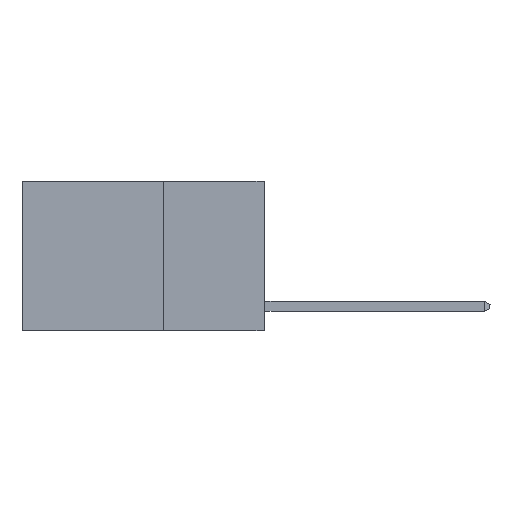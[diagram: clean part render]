
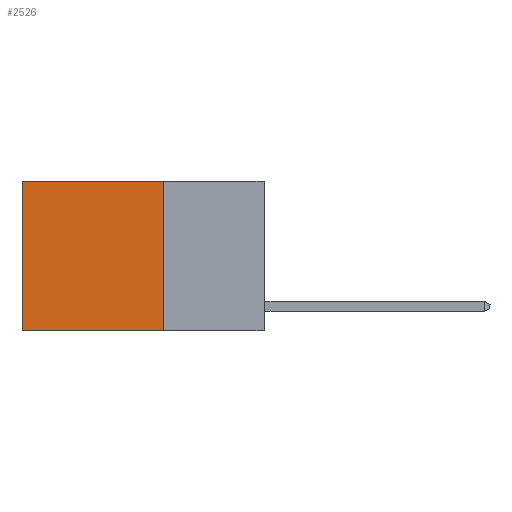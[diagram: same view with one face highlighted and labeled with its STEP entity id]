
A CAD part, left-side view. The second image highlights one B-rep face of the part: STEP entity #2526.
In plain terms, the highlighted planar face has unit normal (-1, 0, 0).
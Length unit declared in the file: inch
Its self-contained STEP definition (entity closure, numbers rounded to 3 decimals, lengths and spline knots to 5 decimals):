
#67 = PLANE ( 'NONE',  #14934 ) ;
#180 = VECTOR ( 'NONE', #2804, 39.37008 ) ;
#997 = CARTESIAN_POINT ( 'NONE',  ( 0.2625, 0.25, 0. ) ) ;
#2526 = ADVANCED_FACE ( 'NONE', ( #22917 ), #67, .F. ) ;
#2804 = DIRECTION ( 'NONE',  ( 0., 0., -1. ) ) ;
#2872 = ORIENTED_EDGE ( 'NONE', *, *, #22839, .F. ) ;
#3686 = DIRECTION ( 'NONE',  ( 0., 0., -1. ) ) ;
#4414 = CARTESIAN_POINT ( 'NONE',  ( 0.2625, 0.6, -0.37 ) ) ;
#4591 = EDGE_LOOP ( 'NONE', ( #13595, #2872, #7528, #22480 ) ) ;
#4717 = CARTESIAN_POINT ( 'NONE',  ( 0.2625, 0.25, -0.37 ) ) ;
#4904 = VECTOR ( 'NONE', #19980, 39.37008 ) ;
#5518 = LINE ( 'NONE', #997, #180 ) ;
#5565 = VECTOR ( 'NONE', #17342, 39.37008 ) ;
#6253 = LINE ( 'NONE', #21526, #19603 ) ;
#6656 = EDGE_CURVE ( 'NONE', #20534, #10073, #15682, .T. ) ;
#7018 = DIRECTION ( 'NONE',  ( 0., 0., -1. ) ) ;
#7486 = VERTEX_POINT ( 'NONE', #4414 ) ;
#7528 = ORIENTED_EDGE ( 'NONE', *, *, #12816, .F. ) ;
#9021 = CARTESIAN_POINT ( 'NONE',  ( 0.2625, 0.25, -0.37 ) ) ;
#9316 = EDGE_CURVE ( 'NONE', #10073, #7486, #6253, .T. ) ;
#10073 = VERTEX_POINT ( 'NONE', #21808 ) ;
#12684 = CARTESIAN_POINT ( 'NONE',  ( 0.2625, 0.25, 0. ) ) ;
#12816 = EDGE_CURVE ( 'NONE', #20534, #14226, #5518, .T. ) ;
#13595 = ORIENTED_EDGE ( 'NONE', *, *, #9316, .T. ) ;
#14226 = VERTEX_POINT ( 'NONE', #9021 ) ;
#14516 = DIRECTION ( 'NONE',  ( 1., 0., 0. ) ) ;
#14545 = CARTESIAN_POINT ( 'NONE',  ( 0.2625, 0.25, 0. ) ) ;
#14934 = AXIS2_PLACEMENT_3D ( 'NONE', #12684, #14516, #3686 ) ;
#15682 = LINE ( 'NONE', #21699, #4904 ) ;
#17342 = DIRECTION ( 'NONE',  ( 0., 1., 0. ) ) ;
#19603 = VECTOR ( 'NONE', #7018, 39.37008 ) ;
#19980 = DIRECTION ( 'NONE',  ( 0., 1., 0. ) ) ;
#20036 = LINE ( 'NONE', #4717, #5565 ) ;
#20534 = VERTEX_POINT ( 'NONE', #14545 ) ;
#21526 = CARTESIAN_POINT ( 'NONE',  ( 0.2625, 0.6, 0. ) ) ;
#21699 = CARTESIAN_POINT ( 'NONE',  ( 0.2625, 0.25, 0. ) ) ;
#21808 = CARTESIAN_POINT ( 'NONE',  ( 0.2625, 0.6, 0. ) ) ;
#22480 = ORIENTED_EDGE ( 'NONE', *, *, #6656, .T. ) ;
#22839 = EDGE_CURVE ( 'NONE', #14226, #7486, #20036, .T. ) ;
#22917 = FACE_OUTER_BOUND ( 'NONE', #4591, .T. ) ;
